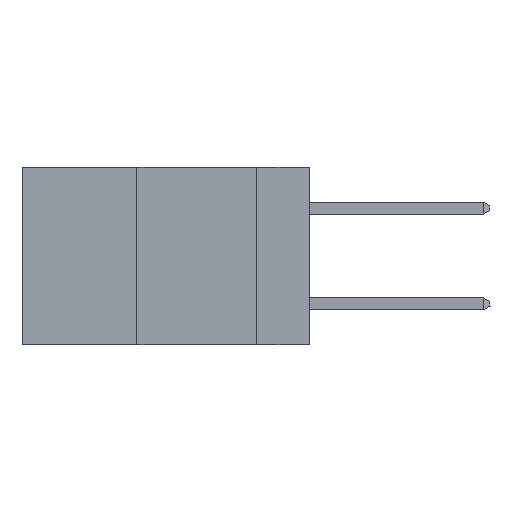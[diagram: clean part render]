
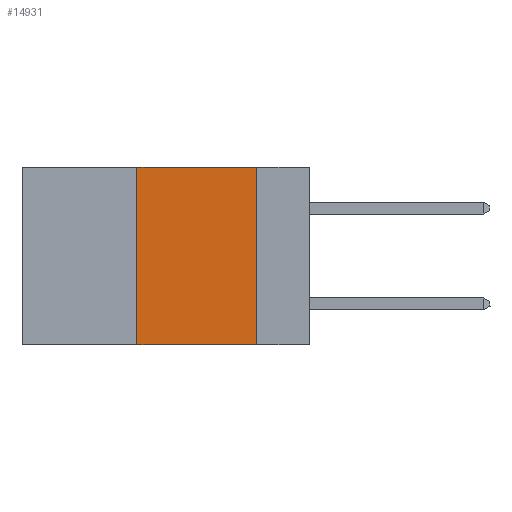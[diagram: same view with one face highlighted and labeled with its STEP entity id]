
A CAD part, left-side view. The second image highlights one B-rep face of the part: STEP entity #14931.
In plain terms, the highlighted planar face has unit normal (-1, 0, 0).
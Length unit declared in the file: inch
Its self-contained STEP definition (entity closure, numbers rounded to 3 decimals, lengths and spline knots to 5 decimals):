
#1022 = VECTOR ( 'NONE', #19087, 39.37008 ) ;
#1155 = EDGE_LOOP ( 'NONE', ( #9248, #7699, #19302, #19093 ) ) ;
#1376 = LINE ( 'NONE', #3416, #14461 ) ;
#2360 = EDGE_CURVE ( 'NONE', #11666, #5845, #14929, .T. ) ;
#3416 = CARTESIAN_POINT ( 'NONE',  ( 0., 0.11, 0. ) ) ;
#3625 = VERTEX_POINT ( 'NONE', #14095 ) ;
#5845 = VERTEX_POINT ( 'NONE', #19078 ) ;
#5956 = EDGE_CURVE ( 'NONE', #11666, #12807, #21619, .T. ) ;
#7699 = ORIENTED_EDGE ( 'NONE', *, *, #13956, .F. ) ;
#8781 = VECTOR ( 'NONE', #12155, 39.37008 ) ;
#8854 = CARTESIAN_POINT ( 'NONE',  ( 0., 0.6, 0. ) ) ;
#8903 = CARTESIAN_POINT ( 'NONE',  ( 0., 0.36, 0. ) ) ;
#9248 = ORIENTED_EDGE ( 'NONE', *, *, #15805, .F. ) ;
#10156 = AXIS2_PLACEMENT_3D ( 'NONE', #21872, #13046, #11469 ) ;
#10386 = DIRECTION ( 'NONE',  ( 0., -1., 0. ) ) ;
#10476 = LINE ( 'NONE', #8854, #11812 ) ;
#10690 = CARTESIAN_POINT ( 'NONE',  ( 0., 0.36, -0.37 ) ) ;
#11469 = DIRECTION ( 'NONE',  ( 0., 0., -1. ) ) ;
#11666 = VERTEX_POINT ( 'NONE', #10690 ) ;
#11812 = VECTOR ( 'NONE', #10386, 39.37008 ) ;
#12155 = DIRECTION ( 'NONE',  ( 0., 0., 1. ) ) ;
#12807 = VERTEX_POINT ( 'NONE', #21375 ) ;
#13046 = DIRECTION ( 'NONE',  ( 1., 0., 0. ) ) ;
#13711 = DIRECTION ( 'NONE',  ( 0., 0., -1. ) ) ;
#13956 = EDGE_CURVE ( 'NONE', #12807, #3625, #10476, .T. ) ;
#14095 = CARTESIAN_POINT ( 'NONE',  ( 0., 0.11, 0. ) ) ;
#14461 = VECTOR ( 'NONE', #13711, 39.37008 ) ;
#14511 = FACE_OUTER_BOUND ( 'NONE', #1155, .T. ) ;
#14751 = PLANE ( 'NONE',  #10156 ) ;
#14929 = LINE ( 'NONE', #17297, #1022 ) ;
#14931 = ADVANCED_FACE ( 'NONE', ( #14511 ), #14751, .F. ) ;
#15805 = EDGE_CURVE ( 'NONE', #3625, #5845, #1376, .T. ) ;
#17297 = CARTESIAN_POINT ( 'NONE',  ( 0., 0.6, -0.37 ) ) ;
#19078 = CARTESIAN_POINT ( 'NONE',  ( 0., 0.11, -0.37 ) ) ;
#19087 = DIRECTION ( 'NONE',  ( 0., -1., 0. ) ) ;
#19093 = ORIENTED_EDGE ( 'NONE', *, *, #2360, .T. ) ;
#19302 = ORIENTED_EDGE ( 'NONE', *, *, #5956, .F. ) ;
#21375 = CARTESIAN_POINT ( 'NONE',  ( 0., 0.36, 0. ) ) ;
#21619 = LINE ( 'NONE', #8903, #8781 ) ;
#21872 = CARTESIAN_POINT ( 'NONE',  ( 0., 0.6, 0. ) ) ;
